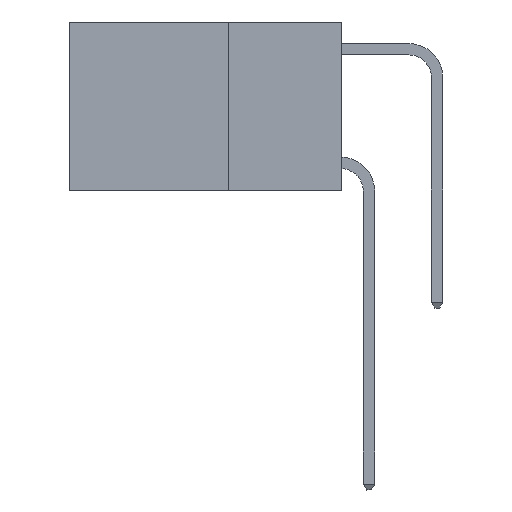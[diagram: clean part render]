
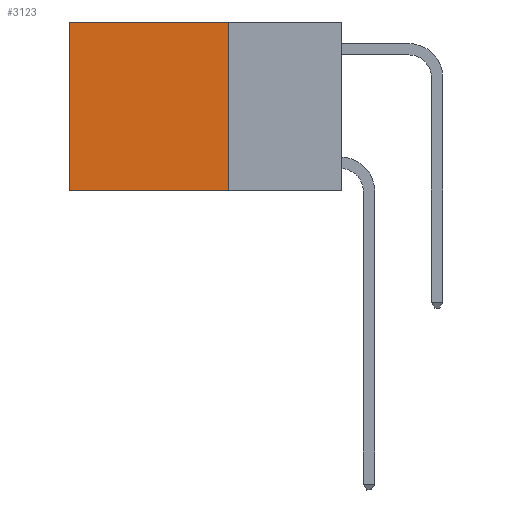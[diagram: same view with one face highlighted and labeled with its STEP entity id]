
A CAD part, left-side view. The second image highlights one B-rep face of the part: STEP entity #3123.
In plain terms, the highlighted planar face has unit normal (-1, 0, 0).
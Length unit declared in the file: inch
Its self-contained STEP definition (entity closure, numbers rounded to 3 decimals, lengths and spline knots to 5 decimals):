
#577 = VERTEX_POINT ( 'NONE', #14842 ) ;
#839 = PLANE ( 'NONE',  #7315 ) ;
#1522 = VECTOR ( 'NONE', #14590, 39.37008 ) ;
#2122 = ORIENTED_EDGE ( 'NONE', *, *, #12516, .F. ) ;
#2876 = CARTESIAN_POINT ( 'NONE',  ( 0.2625, 0.25, -0.37 ) ) ;
#3123 = ADVANCED_FACE ( 'NONE', ( #17195 ), #839, .F. ) ;
#4039 = EDGE_CURVE ( 'NONE', #10637, #18386, #12163, .T. ) ;
#4303 = CARTESIAN_POINT ( 'NONE',  ( 0.2625, 0.25, 0. ) ) ;
#4499 = CARTESIAN_POINT ( 'NONE',  ( 0.2625, 0.6, -0.37 ) ) ;
#4578 = ORIENTED_EDGE ( 'NONE', *, *, #6686, .T. ) ;
#5757 = DIRECTION ( 'NONE',  ( 0., 0., -1. ) ) ;
#6686 = EDGE_CURVE ( 'NONE', #577, #15187, #9015, .T. ) ;
#7315 = AXIS2_PLACEMENT_3D ( 'NONE', #14018, #9893, #18550 ) ;
#7390 = LINE ( 'NONE', #2876, #12923 ) ;
#8139 = CARTESIAN_POINT ( 'NONE',  ( 0.2625, 0.25, -0.37 ) ) ;
#8225 = VECTOR ( 'NONE', #13236, 39.37008 ) ;
#9015 = LINE ( 'NONE', #17780, #13539 ) ;
#9893 = DIRECTION ( 'NONE',  ( 1., 0., 0. ) ) ;
#10081 = LINE ( 'NONE', #4303, #1522 ) ;
#10637 = VERTEX_POINT ( 'NONE', #16007 ) ;
#12163 = LINE ( 'NONE', #18026, #8225 ) ;
#12516 = EDGE_CURVE ( 'NONE', #18386, #15187, #7390, .T. ) ;
#12923 = VECTOR ( 'NONE', #17678, 39.37008 ) ;
#13236 = DIRECTION ( 'NONE',  ( 0., 0., -1. ) ) ;
#13539 = VECTOR ( 'NONE', #5757, 39.37008 ) ;
#14018 = CARTESIAN_POINT ( 'NONE',  ( 0.2625, 0.25, 0. ) ) ;
#14077 = ORIENTED_EDGE ( 'NONE', *, *, #15506, .T. ) ;
#14590 = DIRECTION ( 'NONE',  ( 0., 1., 0. ) ) ;
#14842 = CARTESIAN_POINT ( 'NONE',  ( 0.2625, 0.6, 0. ) ) ;
#15025 = ORIENTED_EDGE ( 'NONE', *, *, #4039, .F. ) ;
#15187 = VERTEX_POINT ( 'NONE', #4499 ) ;
#15382 = EDGE_LOOP ( 'NONE', ( #4578, #2122, #15025, #14077 ) ) ;
#15506 = EDGE_CURVE ( 'NONE', #10637, #577, #10081, .T. ) ;
#16007 = CARTESIAN_POINT ( 'NONE',  ( 0.2625, 0.25, 0. ) ) ;
#17195 = FACE_OUTER_BOUND ( 'NONE', #15382, .T. ) ;
#17678 = DIRECTION ( 'NONE',  ( 0., 1., 0. ) ) ;
#17780 = CARTESIAN_POINT ( 'NONE',  ( 0.2625, 0.6, 0. ) ) ;
#18026 = CARTESIAN_POINT ( 'NONE',  ( 0.2625, 0.25, 0. ) ) ;
#18386 = VERTEX_POINT ( 'NONE', #8139 ) ;
#18550 = DIRECTION ( 'NONE',  ( 0., 0., -1. ) ) ;
